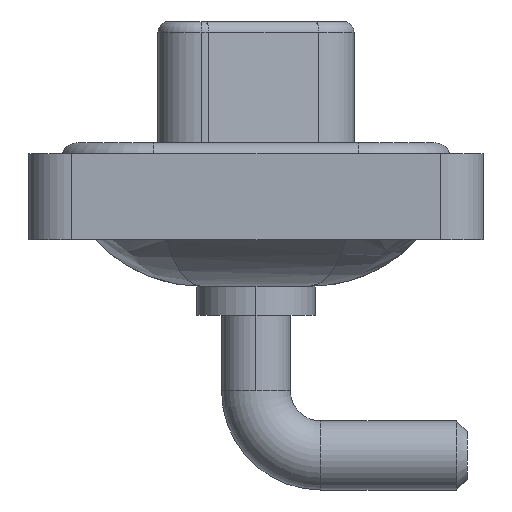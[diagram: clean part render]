
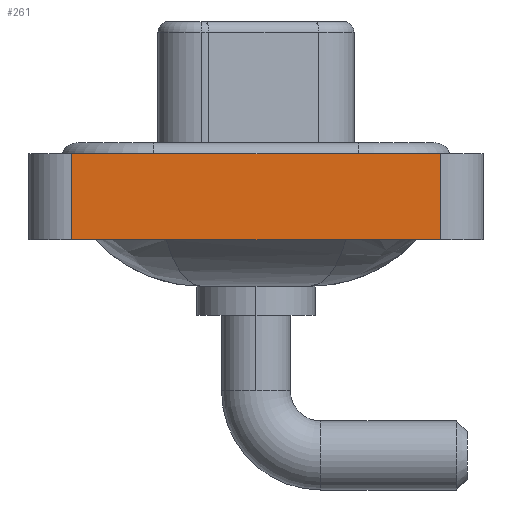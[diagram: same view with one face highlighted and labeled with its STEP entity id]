
A CAD part, left-side view. The second image highlights one B-rep face of the part: STEP entity #261.
In plain terms, the highlighted planar face has unit normal (-1, 0, 0).
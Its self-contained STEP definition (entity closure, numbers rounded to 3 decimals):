
#97 = ORIENTED_EDGE ( 'NONE', *, *, #13134, .F. ) ;
#261 = ADVANCED_FACE ( 'NONE', ( #9162 ), #2512, .T. ) ;
#740 = VERTEX_POINT ( 'NONE', #12678 ) ;
#1192 = LINE ( 'NONE', #10944, #15990 ) ;
#1275 = EDGE_CURVE ( 'NONE', #7815, #17888, #7901, .T. ) ;
#1523 = DIRECTION ( 'NONE',  ( 0., -1., 0. ) ) ;
#1927 = CARTESIAN_POINT ( 'NONE',  ( -7.35, -8.55, 0.4 ) ) ;
#2512 = PLANE ( 'NONE',  #6663 ) ;
#2901 = CARTESIAN_POINT ( 'NONE',  ( -7.35, -8.55, -3.6 ) ) ;
#4323 = CARTESIAN_POINT ( 'NONE',  ( -7.35, -8.55, -3.6 ) ) ;
#4843 = VECTOR ( 'NONE', #1523, 1000. ) ;
#5469 = VECTOR ( 'NONE', #16208, 1000. ) ;
#6500 = DIRECTION ( 'NONE',  ( 0., 0., 1. ) ) ;
#6627 = DIRECTION ( 'NONE',  ( 0., 0., 1. ) ) ;
#6663 = AXIS2_PLACEMENT_3D ( 'NONE', #10890, #14722, #6627 ) ;
#6734 = CARTESIAN_POINT ( 'NONE',  ( -7.35, -8.55, -3.6 ) ) ;
#7315 = VERTEX_POINT ( 'NONE', #8313 ) ;
#7815 = VERTEX_POINT ( 'NONE', #4323 ) ;
#7901 = LINE ( 'NONE', #6734, #5469 ) ;
#8123 = LINE ( 'NONE', #2901, #4843 ) ;
#8313 = CARTESIAN_POINT ( 'NONE',  ( -7.35, 8.55, 0.4 ) ) ;
#9162 = FACE_OUTER_BOUND ( 'NONE', #12851, .T. ) ;
#10890 = CARTESIAN_POINT ( 'NONE',  ( -7.35, -8.55, -3.6 ) ) ;
#10944 = CARTESIAN_POINT ( 'NONE',  ( -7.35, 8.55, -3.6 ) ) ;
#11201 = EDGE_CURVE ( 'NONE', #7315, #17888, #14503, .T. ) ;
#12678 = CARTESIAN_POINT ( 'NONE',  ( -7.35, 8.55, -3.6 ) ) ;
#12851 = EDGE_LOOP ( 'NONE', ( #14895, #15597, #97, #17101 ) ) ;
#13134 = EDGE_CURVE ( 'NONE', #740, #7315, #1192, .T. ) ;
#14503 = LINE ( 'NONE', #1927, #15400 ) ;
#14722 = DIRECTION ( 'NONE',  ( -1., 0., 0. ) ) ;
#14825 = EDGE_CURVE ( 'NONE', #740, #7815, #8123, .T. ) ;
#14895 = ORIENTED_EDGE ( 'NONE', *, *, #1275, .T. ) ;
#15400 = VECTOR ( 'NONE', #17069, 1000. ) ;
#15597 = ORIENTED_EDGE ( 'NONE', *, *, #11201, .F. ) ;
#15990 = VECTOR ( 'NONE', #6500, 1000. ) ;
#16208 = DIRECTION ( 'NONE',  ( 0., 0., 1. ) ) ;
#17069 = DIRECTION ( 'NONE',  ( 0., -1., 0. ) ) ;
#17101 = ORIENTED_EDGE ( 'NONE', *, *, #14825, .T. ) ;
#17888 = VERTEX_POINT ( 'NONE', #18058 ) ;
#18058 = CARTESIAN_POINT ( 'NONE',  ( -7.35, -8.55, 0.4 ) ) ;
